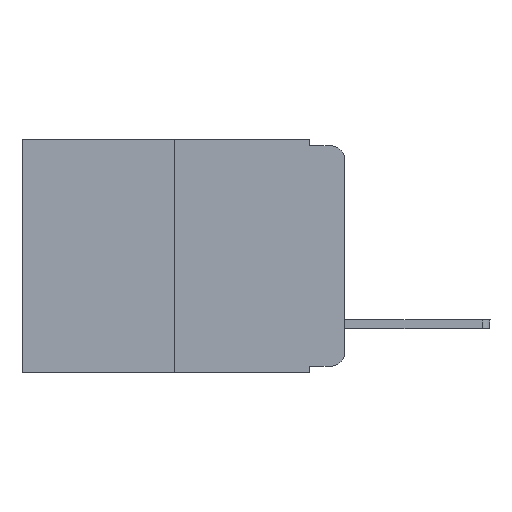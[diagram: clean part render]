
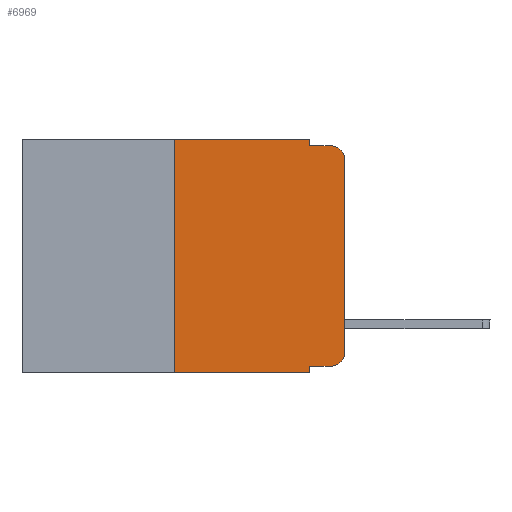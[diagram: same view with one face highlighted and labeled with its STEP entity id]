
A CAD part, left-side view. The second image highlights one B-rep face of the part: STEP entity #6969.
In plain terms, the highlighted planar face has unit normal (-1, 0, 0).
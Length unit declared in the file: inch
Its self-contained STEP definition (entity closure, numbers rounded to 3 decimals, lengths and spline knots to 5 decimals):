
#186 = VERTEX_POINT ( 'NONE', #10996 ) ;
#675 = ORIENTED_EDGE ( 'NONE', *, *, #9524, .T. ) ;
#870 = EDGE_CURVE ( 'NONE', #17048, #186, #3782, .T. ) ;
#1264 = CARTESIAN_POINT ( 'NONE',  ( 0., 0.02, -0.333 ) ) ;
#1574 = VERTEX_POINT ( 'NONE', #10388 ) ;
#1589 = VECTOR ( 'NONE', #18624, 39.37008 ) ;
#2042 = LINE ( 'NONE', #18139, #20037 ) ;
#2113 = CARTESIAN_POINT ( 'NONE',  ( 0., 0.051, -0.343 ) ) ;
#2146 = CARTESIAN_POINT ( 'NONE',  ( 0., 0.051, -0.333 ) ) ;
#2239 = DIRECTION ( 'NONE',  ( 1., 0., 0. ) ) ;
#2832 = LINE ( 'NONE', #17864, #19777 ) ;
#3209 = DIRECTION ( 'NONE',  ( 0., 0., -1. ) ) ;
#3782 = LINE ( 'NONE', #19236, #19992 ) ;
#3790 = LINE ( 'NONE', #18821, #7605 ) ;
#3820 = CARTESIAN_POINT ( 'NONE',  ( 0., 0.051, -0.333 ) ) ;
#4028 = CARTESIAN_POINT ( 'NONE',  ( 0., 0.473, 0. ) ) ;
#4258 = VERTEX_POINT ( 'NONE', #6508 ) ;
#4521 = VERTEX_POINT ( 'NONE', #17066 ) ;
#4644 = ORIENTED_EDGE ( 'NONE', *, *, #870, .T. ) ;
#4671 = DIRECTION ( 'NONE',  ( 0., 0., -1. ) ) ;
#4745 = ORIENTED_EDGE ( 'NONE', *, *, #4862, .T. ) ;
#4797 = VERTEX_POINT ( 'NONE', #2113 ) ;
#4862 = EDGE_CURVE ( 'NONE', #18621, #12600, #17009, .T. ) ;
#5077 = LINE ( 'NONE', #6215, #16433 ) ;
#5577 = CIRCLE ( 'NONE', #20711, 0.02 ) ;
#5967 = EDGE_CURVE ( 'NONE', #4521, #15797, #2042, .T. ) ;
#6215 = CARTESIAN_POINT ( 'NONE',  ( 0., 0.051, 0. ) ) ;
#6508 = CARTESIAN_POINT ( 'NONE',  ( 0., 0.25, 0. ) ) ;
#6969 = ADVANCED_FACE ( 'NONE', ( #14766 ), #19285, .F. ) ;
#7402 = DIRECTION ( 'NONE',  ( -1., 0., 0. ) ) ;
#7494 = CARTESIAN_POINT ( 'NONE',  ( 0., 0.473, 0. ) ) ;
#7519 = DIRECTION ( 'NONE',  ( 0., 0., 1. ) ) ;
#7605 = VECTOR ( 'NONE', #13773, 39.37008 ) ;
#8080 = AXIS2_PLACEMENT_3D ( 'NONE', #17210, #18820, #3209 ) ;
#8159 = CARTESIAN_POINT ( 'NONE',  ( 0., 0.25, 0. ) ) ;
#8291 = DIRECTION ( 'NONE',  ( 0., 0., 1. ) ) ;
#8354 = ORIENTED_EDGE ( 'NONE', *, *, #10412, .F. ) ;
#9182 = AXIS2_PLACEMENT_3D ( 'NONE', #7494, #2239, #18683 ) ;
#9246 = CARTESIAN_POINT ( 'NONE',  ( 0., 0., -0.313 ) ) ;
#9478 = ORIENTED_EDGE ( 'NONE', *, *, #14911, .F. ) ;
#9524 = EDGE_CURVE ( 'NONE', #186, #15797, #19780, .T. ) ;
#10019 = EDGE_CURVE ( 'NONE', #1574, #4521, #5077, .T. ) ;
#10388 = CARTESIAN_POINT ( 'NONE',  ( 0., 0.051, 0. ) ) ;
#10412 = EDGE_CURVE ( 'NONE', #18621, #4797, #3790, .T. ) ;
#10467 = VECTOR ( 'NONE', #8291, 39.37008 ) ;
#10484 = VERTEX_POINT ( 'NONE', #20779 ) ;
#10487 = EDGE_CURVE ( 'NONE', #12600, #17048, #5577, .T. ) ;
#10996 = CARTESIAN_POINT ( 'NONE',  ( 0., 0., -0.03 ) ) ;
#11275 = CARTESIAN_POINT ( 'NONE',  ( 0., 0.02, -0.01 ) ) ;
#12150 = DIRECTION ( 'NONE',  ( 0., -1., 0. ) ) ;
#12600 = VERTEX_POINT ( 'NONE', #1264 ) ;
#13773 = DIRECTION ( 'NONE',  ( 0., 0., -1. ) ) ;
#13801 = ORIENTED_EDGE ( 'NONE', *, *, #10019, .F. ) ;
#14766 = FACE_OUTER_BOUND ( 'NONE', #18361, .T. ) ;
#14836 = ORIENTED_EDGE ( 'NONE', *, *, #10487, .T. ) ;
#14911 = EDGE_CURVE ( 'NONE', #4258, #1574, #17790, .T. ) ;
#15797 = VERTEX_POINT ( 'NONE', #11275 ) ;
#15948 = CARTESIAN_POINT ( 'NONE',  ( 0., 0.02, -0.313 ) ) ;
#16063 = DIRECTION ( 'NONE',  ( 0., -1., 0. ) ) ;
#16142 = LINE ( 'NONE', #8159, #10467 ) ;
#16433 = VECTOR ( 'NONE', #4671, 39.37008 ) ;
#16623 = DIRECTION ( 'NONE',  ( 0., -1., 0. ) ) ;
#17009 = LINE ( 'NONE', #3820, #18552 ) ;
#17048 = VERTEX_POINT ( 'NONE', #9246 ) ;
#17066 = CARTESIAN_POINT ( 'NONE',  ( 0., 0.051, -0.01 ) ) ;
#17210 = CARTESIAN_POINT ( 'NONE',  ( 0., 0.02, -0.03 ) ) ;
#17310 = DIRECTION ( 'NONE',  ( 0., 0., -1. ) ) ;
#17790 = LINE ( 'NONE', #4028, #1589 ) ;
#17864 = CARTESIAN_POINT ( 'NONE',  ( 0., 0.473, -0.343 ) ) ;
#18139 = CARTESIAN_POINT ( 'NONE',  ( 0., 0.051, -0.01 ) ) ;
#18361 = EDGE_LOOP ( 'NONE', ( #4644, #675, #20070, #13801, #9478, #20971, #20731, #8354, #4745, #14836 ) ) ;
#18552 = VECTOR ( 'NONE', #12150, 39.37008 ) ;
#18621 = VERTEX_POINT ( 'NONE', #2146 ) ;
#18624 = DIRECTION ( 'NONE',  ( 0., -1., 0. ) ) ;
#18683 = DIRECTION ( 'NONE',  ( 0., 0., -1. ) ) ;
#18820 = DIRECTION ( 'NONE',  ( -1., 0., 0. ) ) ;
#18821 = CARTESIAN_POINT ( 'NONE',  ( 0., 0.051, 0. ) ) ;
#19236 = CARTESIAN_POINT ( 'NONE',  ( 0., 0., 0. ) ) ;
#19285 = PLANE ( 'NONE',  #9182 ) ;
#19777 = VECTOR ( 'NONE', #16063, 39.37008 ) ;
#19780 = CIRCLE ( 'NONE', #8080, 0.02 ) ;
#19992 = VECTOR ( 'NONE', #7519, 39.37008 ) ;
#20037 = VECTOR ( 'NONE', #16623, 39.37008 ) ;
#20070 = ORIENTED_EDGE ( 'NONE', *, *, #5967, .F. ) ;
#20219 = EDGE_CURVE ( 'NONE', #10484, #4797, #2832, .T. ) ;
#20711 = AXIS2_PLACEMENT_3D ( 'NONE', #15948, #7402, #17310 ) ;
#20731 = ORIENTED_EDGE ( 'NONE', *, *, #20219, .T. ) ;
#20779 = CARTESIAN_POINT ( 'NONE',  ( 0., 0.25, -0.343 ) ) ;
#20971 = ORIENTED_EDGE ( 'NONE', *, *, #21039, .F. ) ;
#21039 = EDGE_CURVE ( 'NONE', #10484, #4258, #16142, .T. ) ;
